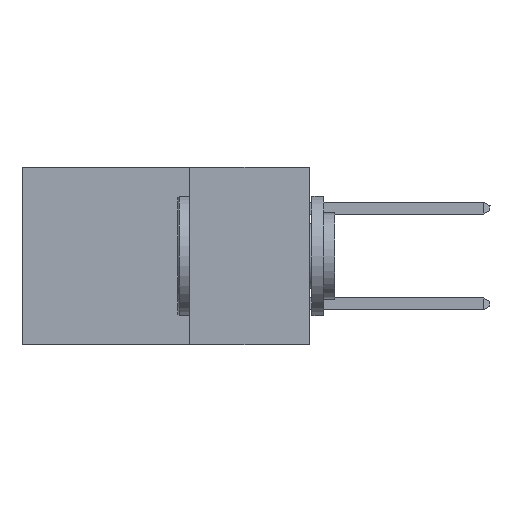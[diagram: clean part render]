
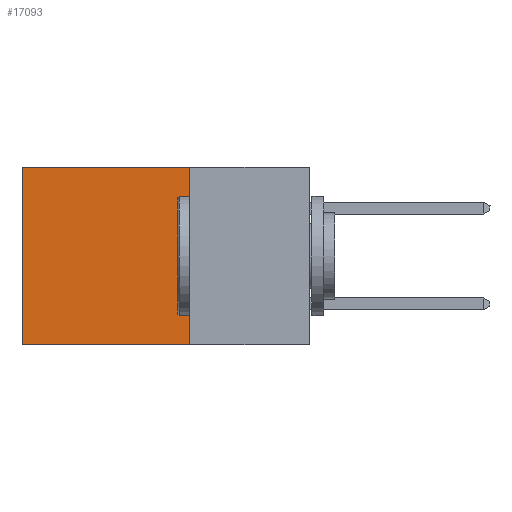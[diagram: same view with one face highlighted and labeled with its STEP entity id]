
A CAD part, left-side view. The second image highlights one B-rep face of the part: STEP entity #17093.
In plain terms, the highlighted planar face has unit normal (-1, 0, 0).
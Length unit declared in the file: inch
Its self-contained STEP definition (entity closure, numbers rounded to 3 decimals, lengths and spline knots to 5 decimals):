
#584 = DIRECTION ( 'NONE',  ( 0., 1., 0. ) ) ;
#1047 = ORIENTED_EDGE ( 'NONE', *, *, #21179, .T. ) ;
#1088 = LINE ( 'NONE', #1618, #5353 ) ;
#1179 = FACE_OUTER_BOUND ( 'NONE', #6675, .T. ) ;
#1275 = PLANE ( 'NONE',  #15061 ) ;
#1358 = DIRECTION ( 'NONE',  ( 1., 0., 0. ) ) ;
#1618 = CARTESIAN_POINT ( 'NONE',  ( 0.2875, 0.6, 0. ) ) ;
#1876 = VERTEX_POINT ( 'NONE', #19364 ) ;
#3099 = ORIENTED_EDGE ( 'NONE', *, *, #19947, .F. ) ;
#3882 = VERTEX_POINT ( 'NONE', #13539 ) ;
#3968 = DIRECTION ( 'NONE',  ( 0., 0., -1. ) ) ;
#4869 = ORIENTED_EDGE ( 'NONE', *, *, #12249, .T. ) ;
#5353 = VECTOR ( 'NONE', #14200, 39.37008 ) ;
#6013 = LINE ( 'NONE', #21727, #19612 ) ;
#6675 = EDGE_LOOP ( 'NONE', ( #1047, #3099, #13096, #4869 ) ) ;
#7894 = VECTOR ( 'NONE', #584, 39.37008 ) ;
#10750 = VERTEX_POINT ( 'NONE', #12427 ) ;
#11455 = CARTESIAN_POINT ( 'NONE',  ( 0.2875, 0.25, -0.37 ) ) ;
#11803 = CARTESIAN_POINT ( 'NONE',  ( 0.2875, 0.25, 0. ) ) ;
#12249 = EDGE_CURVE ( 'NONE', #10750, #16702, #23012, .T. ) ;
#12427 = CARTESIAN_POINT ( 'NONE',  ( 0.2875, 0.25, 0. ) ) ;
#13096 = ORIENTED_EDGE ( 'NONE', *, *, #18692, .F. ) ;
#13539 = CARTESIAN_POINT ( 'NONE',  ( 0.2875, 0.6, -0.37 ) ) ;
#13868 = DIRECTION ( 'NONE',  ( 0., 0., -1. ) ) ;
#14200 = DIRECTION ( 'NONE',  ( 0., 0., -1. ) ) ;
#14587 = CARTESIAN_POINT ( 'NONE',  ( 0.2875, 0.6, 0. ) ) ;
#15061 = AXIS2_PLACEMENT_3D ( 'NONE', #20927, #1358, #13868 ) ;
#16702 = VERTEX_POINT ( 'NONE', #14587 ) ;
#17093 = ADVANCED_FACE ( 'NONE', ( #1179 ), #1275, .F. ) ;
#18392 = VECTOR ( 'NONE', #20649, 39.37008 ) ;
#18692 = EDGE_CURVE ( 'NONE', #10750, #1876, #6013, .T. ) ;
#19364 = CARTESIAN_POINT ( 'NONE',  ( 0.2875, 0.25, -0.37 ) ) ;
#19612 = VECTOR ( 'NONE', #3968, 39.37008 ) ;
#19947 = EDGE_CURVE ( 'NONE', #1876, #3882, #21438, .T. ) ;
#20649 = DIRECTION ( 'NONE',  ( 0., 1., 0. ) ) ;
#20927 = CARTESIAN_POINT ( 'NONE',  ( 0.2875, 0.25, 0. ) ) ;
#21179 = EDGE_CURVE ( 'NONE', #16702, #3882, #1088, .T. ) ;
#21438 = LINE ( 'NONE', #11455, #7894 ) ;
#21727 = CARTESIAN_POINT ( 'NONE',  ( 0.2875, 0.25, 0. ) ) ;
#23012 = LINE ( 'NONE', #11803, #18392 ) ;
